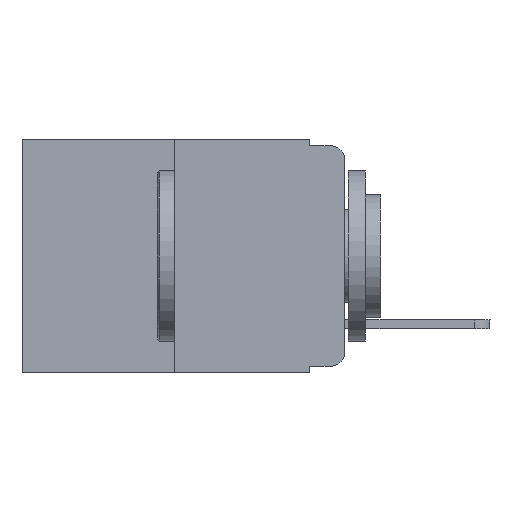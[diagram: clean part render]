
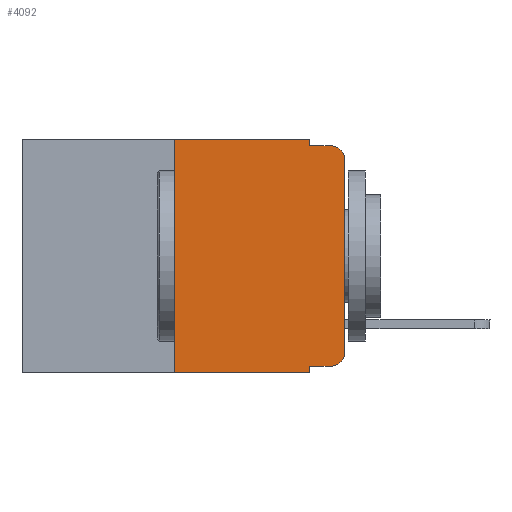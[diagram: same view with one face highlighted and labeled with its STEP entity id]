
A CAD part, left-side view. The second image highlights one B-rep face of the part: STEP entity #4092.
In plain terms, the highlighted planar face has unit normal (-1, 0, 0).
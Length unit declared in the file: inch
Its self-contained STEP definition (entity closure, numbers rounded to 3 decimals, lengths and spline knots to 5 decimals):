
#89 = ORIENTED_EDGE ( 'NONE', *, *, #15491, .F. ) ;
#992 = DIRECTION ( 'NONE',  ( 1., 0., 0. ) ) ;
#1069 = VERTEX_POINT ( 'NONE', #6872 ) ;
#1593 = EDGE_LOOP ( 'NONE', ( #13879, #12778, #89, #16581, #2395, #6042, #4535, #14674, #16587, #16227 ) ) ;
#1655 = EDGE_CURVE ( 'NONE', #1069, #2258, #12120, .T. ) ;
#2258 = VERTEX_POINT ( 'NONE', #11048 ) ;
#2296 = CARTESIAN_POINT ( 'NONE',  ( 0., 0.051, -0.01 ) ) ;
#2395 = ORIENTED_EDGE ( 'NONE', *, *, #3600, .F. ) ;
#2651 = LINE ( 'NONE', #13466, #10013 ) ;
#2786 = CARTESIAN_POINT ( 'NONE',  ( 0., 0., 0. ) ) ;
#2951 = DIRECTION ( 'NONE',  ( 0., 0., -1. ) ) ;
#3552 = LINE ( 'NONE', #13373, #8187 ) ;
#3600 = EDGE_CURVE ( 'NONE', #8771, #10325, #3552, .T. ) ;
#3606 = DIRECTION ( 'NONE',  ( 0., 0., -1. ) ) ;
#4041 = EDGE_CURVE ( 'NONE', #5515, #8131, #11380, .T. ) ;
#4092 = ADVANCED_FACE ( 'NONE', ( #17255 ), #16084, .F. ) ;
#4308 = EDGE_CURVE ( 'NONE', #7100, #4708, #7906, .T. ) ;
#4535 = ORIENTED_EDGE ( 'NONE', *, *, #9346, .T. ) ;
#4708 = VERTEX_POINT ( 'NONE', #14316 ) ;
#4742 = EDGE_CURVE ( 'NONE', #10325, #11291, #7398, .T. ) ;
#4799 = CARTESIAN_POINT ( 'NONE',  ( 0., 0.473, 0. ) ) ;
#5230 = CARTESIAN_POINT ( 'NONE',  ( 0., 0.25, -0.343 ) ) ;
#5474 = LINE ( 'NONE', #11041, #15569 ) ;
#5515 = VERTEX_POINT ( 'NONE', #5517 ) ;
#5517 = CARTESIAN_POINT ( 'NONE',  ( 0., 0., -0.03 ) ) ;
#5670 = CARTESIAN_POINT ( 'NONE',  ( 0., 0.051, 0. ) ) ;
#6042 = ORIENTED_EDGE ( 'NONE', *, *, #11685, .F. ) ;
#6218 = DIRECTION ( 'NONE',  ( 0., -1., 0. ) ) ;
#6872 = CARTESIAN_POINT ( 'NONE',  ( 0., 0.051, -0.333 ) ) ;
#7100 = VERTEX_POINT ( 'NONE', #14992 ) ;
#7107 = VECTOR ( 'NONE', #17783, 39.37008 ) ;
#7398 = LINE ( 'NONE', #5670, #14188 ) ;
#7648 = CARTESIAN_POINT ( 'NONE',  ( 0., 0.051, 0. ) ) ;
#7890 = AXIS2_PLACEMENT_3D ( 'NONE', #9355, #13438, #13176 ) ;
#7906 = CIRCLE ( 'NONE', #11975, 0.02 ) ;
#8131 = VERTEX_POINT ( 'NONE', #9511 ) ;
#8187 = VECTOR ( 'NONE', #17374, 39.37008 ) ;
#8298 = CARTESIAN_POINT ( 'NONE',  ( 0., 0.25, 0. ) ) ;
#8771 = VERTEX_POINT ( 'NONE', #8298 ) ;
#9061 = CARTESIAN_POINT ( 'NONE',  ( 0., 0.473, -0.343 ) ) ;
#9346 = EDGE_CURVE ( 'NONE', #17550, #2258, #13151, .T. ) ;
#9355 = CARTESIAN_POINT ( 'NONE',  ( 0., 0.02, -0.03 ) ) ;
#9511 = CARTESIAN_POINT ( 'NONE',  ( 0., 0.02, -0.01 ) ) ;
#9936 = AXIS2_PLACEMENT_3D ( 'NONE', #4799, #992, #3606 ) ;
#10013 = VECTOR ( 'NONE', #14912, 39.37008 ) ;
#10064 = DIRECTION ( 'NONE',  ( 0., 0., -1. ) ) ;
#10091 = VECTOR ( 'NONE', #17732, 39.37008 ) ;
#10325 = VERTEX_POINT ( 'NONE', #7648 ) ;
#10432 = VECTOR ( 'NONE', #6218, 39.37008 ) ;
#10661 = DIRECTION ( 'NONE',  ( 0., 0., -1. ) ) ;
#11041 = CARTESIAN_POINT ( 'NONE',  ( 0., 0.051, -0.333 ) ) ;
#11048 = CARTESIAN_POINT ( 'NONE',  ( 0., 0.051, -0.343 ) ) ;
#11291 = VERTEX_POINT ( 'NONE', #13156 ) ;
#11380 = CIRCLE ( 'NONE', #7890, 0.02 ) ;
#11685 = EDGE_CURVE ( 'NONE', #17550, #8771, #2651, .T. ) ;
#11975 = AXIS2_PLACEMENT_3D ( 'NONE', #16969, #12699, #10064 ) ;
#12120 = LINE ( 'NONE', #13757, #13819 ) ;
#12699 = DIRECTION ( 'NONE',  ( -1., 0., 0. ) ) ;
#12778 = ORIENTED_EDGE ( 'NONE', *, *, #4041, .T. ) ;
#13125 = EDGE_CURVE ( 'NONE', #1069, #7100, #5474, .T. ) ;
#13151 = LINE ( 'NONE', #9061, #10432 ) ;
#13156 = CARTESIAN_POINT ( 'NONE',  ( 0., 0.051, -0.01 ) ) ;
#13176 = DIRECTION ( 'NONE',  ( 0., 0., -1. ) ) ;
#13373 = CARTESIAN_POINT ( 'NONE',  ( 0., 0.473, 0. ) ) ;
#13438 = DIRECTION ( 'NONE',  ( -1., 0., 0. ) ) ;
#13466 = CARTESIAN_POINT ( 'NONE',  ( 0., 0.25, 0. ) ) ;
#13757 = CARTESIAN_POINT ( 'NONE',  ( 0., 0.051, 0. ) ) ;
#13819 = VECTOR ( 'NONE', #10661, 39.37008 ) ;
#13879 = ORIENTED_EDGE ( 'NONE', *, *, #17730, .T. ) ;
#14188 = VECTOR ( 'NONE', #2951, 39.37008 ) ;
#14316 = CARTESIAN_POINT ( 'NONE',  ( 0., 0., -0.313 ) ) ;
#14674 = ORIENTED_EDGE ( 'NONE', *, *, #1655, .F. ) ;
#14743 = LINE ( 'NONE', #2296, #10091 ) ;
#14912 = DIRECTION ( 'NONE',  ( 0., 0., 1. ) ) ;
#14992 = CARTESIAN_POINT ( 'NONE',  ( 0., 0.02, -0.333 ) ) ;
#15240 = LINE ( 'NONE', #2786, #7107 ) ;
#15491 = EDGE_CURVE ( 'NONE', #11291, #8131, #14743, .T. ) ;
#15569 = VECTOR ( 'NONE', #16678, 39.37008 ) ;
#16084 = PLANE ( 'NONE',  #9936 ) ;
#16227 = ORIENTED_EDGE ( 'NONE', *, *, #4308, .T. ) ;
#16581 = ORIENTED_EDGE ( 'NONE', *, *, #4742, .F. ) ;
#16587 = ORIENTED_EDGE ( 'NONE', *, *, #13125, .T. ) ;
#16678 = DIRECTION ( 'NONE',  ( 0., -1., 0. ) ) ;
#16969 = CARTESIAN_POINT ( 'NONE',  ( 0., 0.02, -0.313 ) ) ;
#17255 = FACE_OUTER_BOUND ( 'NONE', #1593, .T. ) ;
#17374 = DIRECTION ( 'NONE',  ( 0., -1., 0. ) ) ;
#17550 = VERTEX_POINT ( 'NONE', #5230 ) ;
#17730 = EDGE_CURVE ( 'NONE', #4708, #5515, #15240, .T. ) ;
#17732 = DIRECTION ( 'NONE',  ( 0., -1., 0. ) ) ;
#17783 = DIRECTION ( 'NONE',  ( 0., 0., 1. ) ) ;
